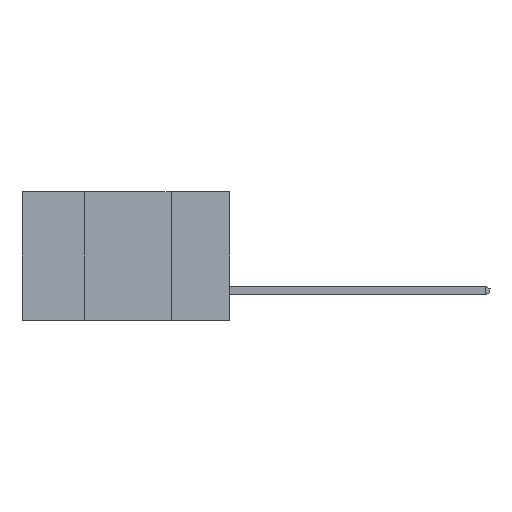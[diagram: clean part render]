
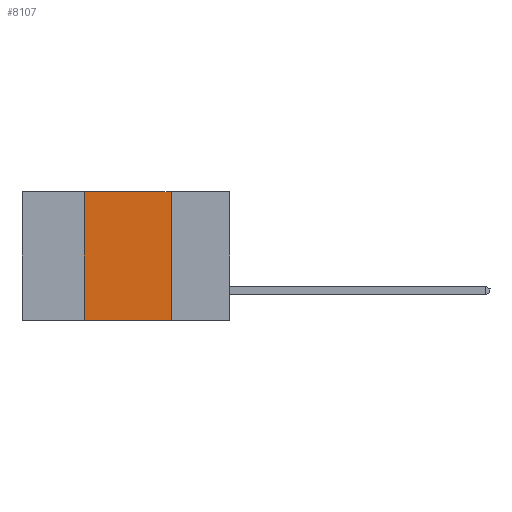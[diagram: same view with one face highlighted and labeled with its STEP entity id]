
A CAD part, left-side view. The second image highlights one B-rep face of the part: STEP entity #8107.
In plain terms, the highlighted planar face has unit normal (-1, 0, 0).
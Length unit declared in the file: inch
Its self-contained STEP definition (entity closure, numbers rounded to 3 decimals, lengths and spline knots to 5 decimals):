
#206 = EDGE_CURVE ( 'NONE', #8201, #6041, #5935, .T. ) ;
#875 = EDGE_CURVE ( 'NONE', #8201, #3178, #2633, .T. ) ;
#1134 = DIRECTION ( 'NONE',  ( 0., 0., 1. ) ) ;
#1406 = EDGE_CURVE ( 'NONE', #3178, #4907, #4594, .T. ) ;
#1633 = PLANE ( 'NONE',  #3193 ) ;
#1790 = CARTESIAN_POINT ( 'NONE',  ( 0., 0.6, -0.37 ) ) ;
#2399 = CARTESIAN_POINT ( 'NONE',  ( 0., 0.42, -0.37 ) ) ;
#2536 = VECTOR ( 'NONE', #6105, 39.37008 ) ;
#2633 = LINE ( 'NONE', #5376, #3974 ) ;
#3019 = EDGE_LOOP ( 'NONE', ( #8423, #8366, #7907, #6084 ) ) ;
#3178 = VERTEX_POINT ( 'NONE', #4728 ) ;
#3193 = AXIS2_PLACEMENT_3D ( 'NONE', #7062, #7646, #8327 ) ;
#3858 = DIRECTION ( 'NONE',  ( 0., -1., 0. ) ) ;
#3970 = LINE ( 'NONE', #5371, #2536 ) ;
#3974 = VECTOR ( 'NONE', #1134, 39.37008 ) ;
#4594 = LINE ( 'NONE', #5148, #7024 ) ;
#4728 = CARTESIAN_POINT ( 'NONE',  ( 0., 0.42, 0. ) ) ;
#4846 = EDGE_CURVE ( 'NONE', #4907, #6041, #3970, .T. ) ;
#4907 = VERTEX_POINT ( 'NONE', #8677 ) ;
#5138 = VECTOR ( 'NONE', #3858, 39.37008 ) ;
#5148 = CARTESIAN_POINT ( 'NONE',  ( 0., 0.6, 0. ) ) ;
#5371 = CARTESIAN_POINT ( 'NONE',  ( 0., 0.17, -0.37 ) ) ;
#5376 = CARTESIAN_POINT ( 'NONE',  ( 0., 0.42, -0.37 ) ) ;
#5935 = LINE ( 'NONE', #1790, #5138 ) ;
#6041 = VERTEX_POINT ( 'NONE', #8735 ) ;
#6084 = ORIENTED_EDGE ( 'NONE', *, *, #206, .T. ) ;
#6105 = DIRECTION ( 'NONE',  ( 0., 0., -1. ) ) ;
#7024 = VECTOR ( 'NONE', #7925, 39.37008 ) ;
#7062 = CARTESIAN_POINT ( 'NONE',  ( 0., 0.6, 0. ) ) ;
#7646 = DIRECTION ( 'NONE',  ( 1., 0., 0. ) ) ;
#7907 = ORIENTED_EDGE ( 'NONE', *, *, #875, .F. ) ;
#7925 = DIRECTION ( 'NONE',  ( 0., -1., 0. ) ) ;
#8107 = ADVANCED_FACE ( 'NONE', ( #8375 ), #1633, .F. ) ;
#8201 = VERTEX_POINT ( 'NONE', #2399 ) ;
#8327 = DIRECTION ( 'NONE',  ( 0., 0., -1. ) ) ;
#8366 = ORIENTED_EDGE ( 'NONE', *, *, #1406, .F. ) ;
#8375 = FACE_OUTER_BOUND ( 'NONE', #3019, .T. ) ;
#8423 = ORIENTED_EDGE ( 'NONE', *, *, #4846, .F. ) ;
#8677 = CARTESIAN_POINT ( 'NONE',  ( 0., 0.17, 0. ) ) ;
#8735 = CARTESIAN_POINT ( 'NONE',  ( 0., 0.17, -0.37 ) ) ;
